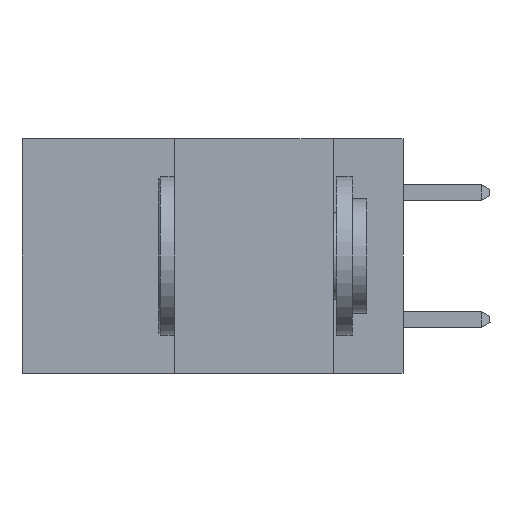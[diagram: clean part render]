
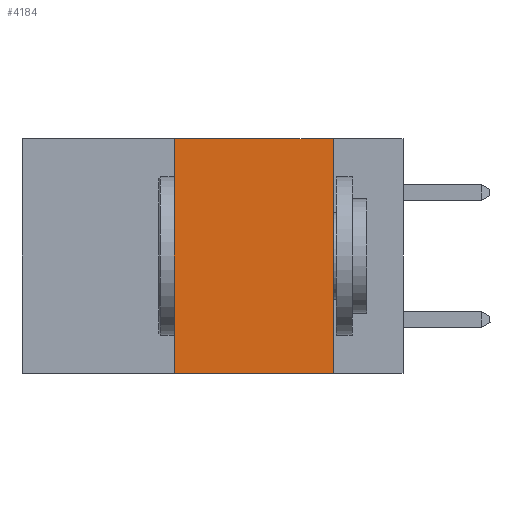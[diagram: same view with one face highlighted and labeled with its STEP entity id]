
A CAD part, left-side view. The second image highlights one B-rep face of the part: STEP entity #4184.
In plain terms, the highlighted planar face has unit normal (-1, 0, 0).
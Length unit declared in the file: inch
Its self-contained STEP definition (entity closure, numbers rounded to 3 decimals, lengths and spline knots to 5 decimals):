
#18 = FACE_OUTER_BOUND ( 'NONE', #14228, .T. ) ;
#366 = LINE ( 'NONE', #10609, #13857 ) ;
#1731 = CARTESIAN_POINT ( 'NONE',  ( 0., 0.36, -0.37 ) ) ;
#1738 = CARTESIAN_POINT ( 'NONE',  ( 0., 0.6, 0. ) ) ;
#1774 = EDGE_CURVE ( 'NONE', #7999, #12588, #18654, .T. ) ;
#2058 = CARTESIAN_POINT ( 'NONE',  ( 0., 0.36, 0. ) ) ;
#2187 = CARTESIAN_POINT ( 'NONE',  ( 0., 0.11, 0. ) ) ;
#2707 = DIRECTION ( 'NONE',  ( 0., 0., 1. ) ) ;
#3138 = DIRECTION ( 'NONE',  ( 0., -1., 0. ) ) ;
#3295 = LINE ( 'NONE', #9424, #10517 ) ;
#4184 = ADVANCED_FACE ( 'NONE', ( #18 ), #15685, .F. ) ;
#4631 = CARTESIAN_POINT ( 'NONE',  ( 0., 0.6, 0. ) ) ;
#5137 = VECTOR ( 'NONE', #3138, 39.37008 ) ;
#6083 = DIRECTION ( 'NONE',  ( 1., 0., 0. ) ) ;
#7999 = VERTEX_POINT ( 'NONE', #2187 ) ;
#8462 = EDGE_CURVE ( 'NONE', #10140, #12588, #3295, .T. ) ;
#9395 = CARTESIAN_POINT ( 'NONE',  ( 0., 0.11, 0. ) ) ;
#9424 = CARTESIAN_POINT ( 'NONE',  ( 0., 0.6, -0.37 ) ) ;
#9503 = DIRECTION ( 'NONE',  ( 0., 0., -1. ) ) ;
#9718 = ORIENTED_EDGE ( 'NONE', *, *, #8462, .T. ) ;
#9780 = DIRECTION ( 'NONE',  ( 0., -1., 0. ) ) ;
#10140 = VERTEX_POINT ( 'NONE', #1731 ) ;
#10517 = VECTOR ( 'NONE', #9780, 39.37008 ) ;
#10609 = CARTESIAN_POINT ( 'NONE',  ( 0., 0.36, 0. ) ) ;
#10714 = ORIENTED_EDGE ( 'NONE', *, *, #19786, .F. ) ;
#11153 = DIRECTION ( 'NONE',  ( 0., 0., -1. ) ) ;
#11635 = ORIENTED_EDGE ( 'NONE', *, *, #1774, .F. ) ;
#11820 = AXIS2_PLACEMENT_3D ( 'NONE', #4631, #6083, #9503 ) ;
#12588 = VERTEX_POINT ( 'NONE', #13556 ) ;
#13141 = LINE ( 'NONE', #1738, #5137 ) ;
#13556 = CARTESIAN_POINT ( 'NONE',  ( 0., 0.11, -0.37 ) ) ;
#13857 = VECTOR ( 'NONE', #2707, 39.37008 ) ;
#14228 = EDGE_LOOP ( 'NONE', ( #11635, #14408, #10714, #9718 ) ) ;
#14408 = ORIENTED_EDGE ( 'NONE', *, *, #18788, .F. ) ;
#15379 = VERTEX_POINT ( 'NONE', #2058 ) ;
#15685 = PLANE ( 'NONE',  #11820 ) ;
#17925 = VECTOR ( 'NONE', #11153, 39.37008 ) ;
#18654 = LINE ( 'NONE', #9395, #17925 ) ;
#18788 = EDGE_CURVE ( 'NONE', #15379, #7999, #13141, .T. ) ;
#19786 = EDGE_CURVE ( 'NONE', #10140, #15379, #366, .T. ) ;
